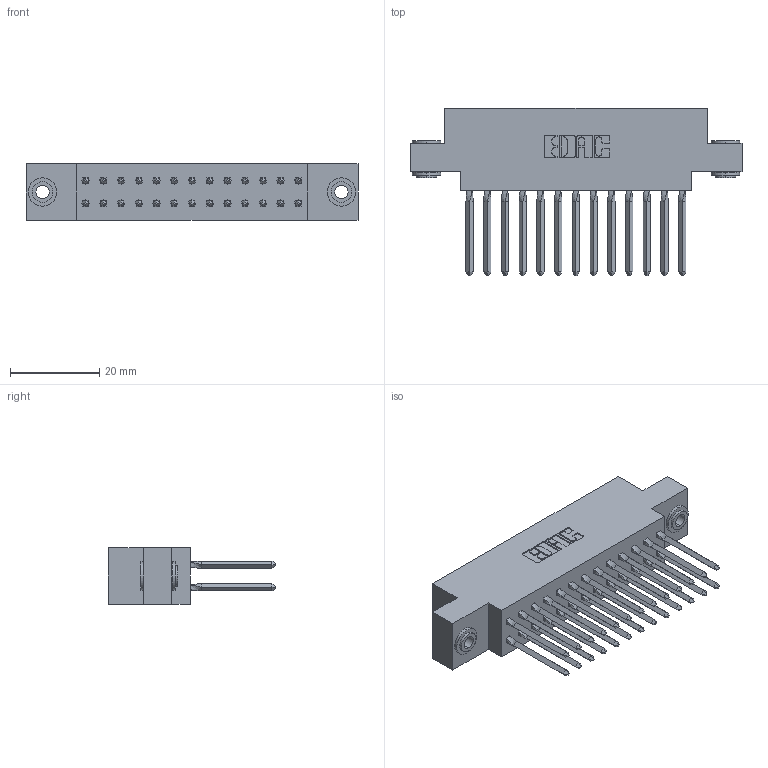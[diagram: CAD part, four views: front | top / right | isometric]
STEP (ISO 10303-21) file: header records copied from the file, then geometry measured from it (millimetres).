
FILE_DESCRIPTION (( 'STEP AP203' ), '1' );
FILE_NAME ('317-026-542-803.STEP', '2020-02-27T18:55:10', ( '' ), ( '' ), 'SwSTEP 2.0', 'SolidWorks 2016', '' );
FILE_SCHEMA (( 'CONFIG_CONTROL_DESIGN' ));
Length unit declared in the file: inch
Products named in the file (4): 317-026-542-803; 345-250-002_345-250-002-102; 317 Part_.156 Dia - TH; 317-290-003_542
Assembly tree (29 placements, depth 2):
  317-026-542-803
    317 Part_.156 Dia - TH
    317-290-003_542  x26
    345-250-002_345-250-002-102  x2
Bounding box: 74.22 x 37.34 x 12.7 mm (x, y, z)
Volume: 11256 mm3; surface area: 14938.2 mm2
Topology: 29 solids, 29 shells, 1622 faces, 4511 edges, 2882 vertices
Faces by surface type: plane 1264, cylinder 246, bspline 104, cone 8
Entity records: 22504 total; most frequent: CARTESIAN_POINT 4140, ORIENTED_EDGE 3796, DIRECTION 3284, EDGE_CURVE 1898, LINE 1704, VECTOR 1704, VERTEX_POINT 1258, AXIS2_PLACEMENT_3D 790
